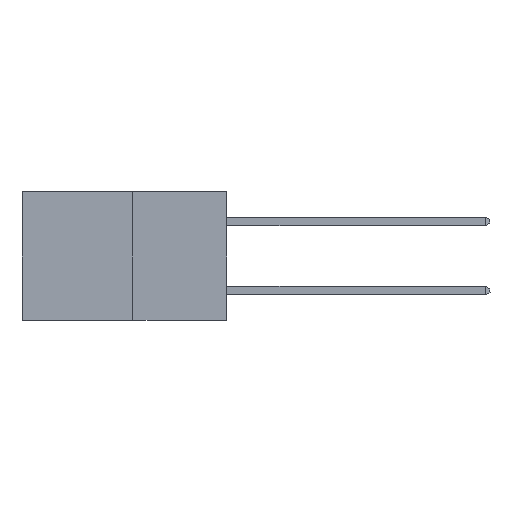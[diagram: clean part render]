
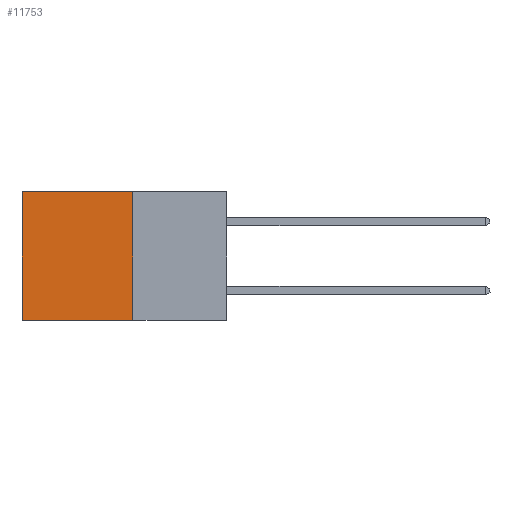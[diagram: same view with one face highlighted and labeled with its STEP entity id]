
A CAD part, left-side view. The second image highlights one B-rep face of the part: STEP entity #11753.
In plain terms, the highlighted planar face has unit normal (-1, 0, 0).
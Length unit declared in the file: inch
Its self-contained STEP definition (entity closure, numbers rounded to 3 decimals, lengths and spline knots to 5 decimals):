
#1422 = CARTESIAN_POINT ( 'NONE',  ( 0.277, 0.27, 0. ) ) ;
#2144 = VERTEX_POINT ( 'NONE', #2676 ) ;
#2676 = CARTESIAN_POINT ( 'NONE',  ( 0.277, 0.27, -0.37 ) ) ;
#2838 = CARTESIAN_POINT ( 'NONE',  ( 0.277, 0.27, -0.37 ) ) ;
#5474 = CARTESIAN_POINT ( 'NONE',  ( 0.277, 0.27, 0. ) ) ;
#6121 = LINE ( 'NONE', #5474, #17231 ) ;
#7060 = DIRECTION ( 'NONE',  ( 0., 0., -1. ) ) ;
#7110 = VERTEX_POINT ( 'NONE', #15569 ) ;
#7726 = DIRECTION ( 'NONE',  ( 0., 1., 0. ) ) ;
#7954 = AXIS2_PLACEMENT_3D ( 'NONE', #26610, #28845, #15498 ) ;
#8548 = LINE ( 'NONE', #2838, #19651 ) ;
#9134 = EDGE_CURVE ( 'NONE', #22795, #2144, #23564, .T. ) ;
#9813 = EDGE_CURVE ( 'NONE', #22795, #7110, #6121, .T. ) ;
#10369 = EDGE_CURVE ( 'NONE', #2144, #14436, #8548, .T. ) ;
#11111 = PLANE ( 'NONE',  #7954 ) ;
#11753 = ADVANCED_FACE ( 'NONE', ( #19557 ), #11111, .F. ) ;
#14436 = VERTEX_POINT ( 'NONE', #19064 ) ;
#14896 = VECTOR ( 'NONE', #7060, 39.37008 ) ;
#15498 = DIRECTION ( 'NONE',  ( 0., 0., -1. ) ) ;
#15569 = CARTESIAN_POINT ( 'NONE',  ( 0.277, 0.59, 0. ) ) ;
#16284 = CARTESIAN_POINT ( 'NONE',  ( 0.277, 0.27, -0.37 ) ) ;
#16858 = ORIENTED_EDGE ( 'NONE', *, *, #10369, .F. ) ;
#17231 = VECTOR ( 'NONE', #7726, 39.37008 ) ;
#17627 = VECTOR ( 'NONE', #23021, 39.37008 ) ;
#18872 = ORIENTED_EDGE ( 'NONE', *, *, #9813, .T. ) ;
#19064 = CARTESIAN_POINT ( 'NONE',  ( 0.277, 0.59, -0.37 ) ) ;
#19557 = FACE_OUTER_BOUND ( 'NONE', #25917, .T. ) ;
#19651 = VECTOR ( 'NONE', #20729, 39.37008 ) ;
#20729 = DIRECTION ( 'NONE',  ( 0., 1., 0. ) ) ;
#20841 = LINE ( 'NONE', #22620, #14896 ) ;
#21050 = ORIENTED_EDGE ( 'NONE', *, *, #9134, .F. ) ;
#22620 = CARTESIAN_POINT ( 'NONE',  ( 0.277, 0.59, -0.37 ) ) ;
#22795 = VERTEX_POINT ( 'NONE', #1422 ) ;
#23021 = DIRECTION ( 'NONE',  ( 0., 0., -1. ) ) ;
#23158 = EDGE_CURVE ( 'NONE', #7110, #14436, #20841, .T. ) ;
#23564 = LINE ( 'NONE', #16284, #17627 ) ;
#24098 = ORIENTED_EDGE ( 'NONE', *, *, #23158, .T. ) ;
#25917 = EDGE_LOOP ( 'NONE', ( #24098, #16858, #21050, #18872 ) ) ;
#26610 = CARTESIAN_POINT ( 'NONE',  ( 0.277, 0.27, -0.37 ) ) ;
#28845 = DIRECTION ( 'NONE',  ( 1., 0., 0. ) ) ;
